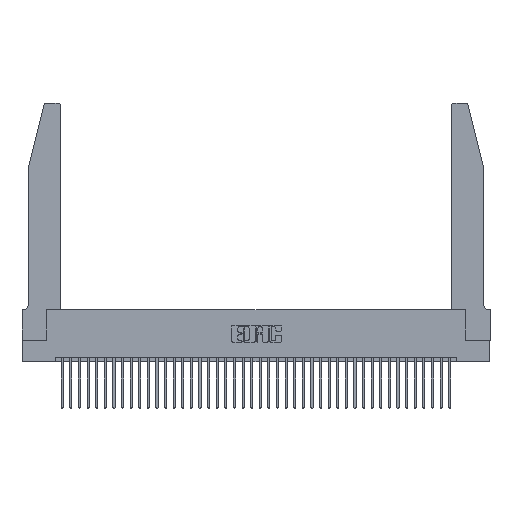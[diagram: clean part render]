
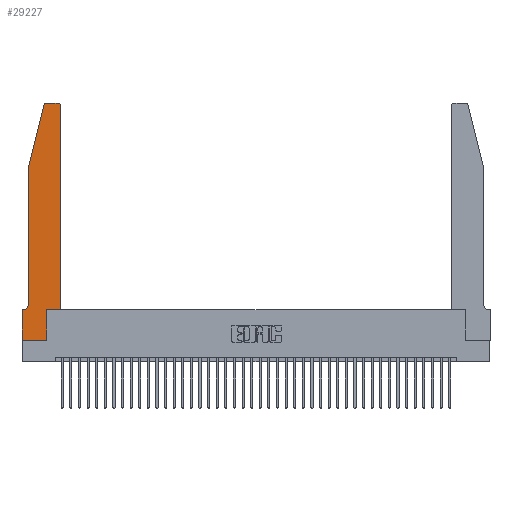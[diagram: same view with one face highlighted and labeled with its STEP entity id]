
A CAD part, top view. The second image highlights one B-rep face of the part: STEP entity #29227.
In plain terms, the highlighted planar face has unit normal (0, 0, 1).
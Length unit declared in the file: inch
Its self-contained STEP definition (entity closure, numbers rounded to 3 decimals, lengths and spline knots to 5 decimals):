
#14 = FACE_OUTER_BOUND ( 'NONE', #1911, .T. ) ;
#633 = VERTEX_POINT ( 'NONE', #12016 ) ;
#730 = LINE ( 'NONE', #8545, #3684 ) ;
#1793 = CARTESIAN_POINT ( 'NONE',  ( 0., 0.35, 0.37 ) ) ;
#1911 = EDGE_LOOP ( 'NONE', ( #19973, #6507, #27655, #17372, #18773, #4992, #32163, #4681, #7863, #10781, #23679, #24845 ) ) ;
#2410 = EDGE_CURVE ( 'NONE', #22411, #9083, #5865, .T. ) ;
#2570 = LINE ( 'NONE', #5586, #18196 ) ;
#2900 = DIRECTION ( 'NONE',  ( 1., 0., 0. ) ) ;
#3074 = CARTESIAN_POINT ( 'NONE',  ( 0., 0., 0.37 ) ) ;
#3684 = VECTOR ( 'NONE', #17501, 39.37008 ) ;
#4178 = VECTOR ( 'NONE', #9894, 39.37008 ) ;
#4681 = ORIENTED_EDGE ( 'NONE', *, *, #6744, .T. ) ;
#4992 = ORIENTED_EDGE ( 'NONE', *, *, #39633, .T. ) ;
#5210 = LINE ( 'NONE', #21528, #19407 ) ;
#5299 = DIRECTION ( 'NONE',  ( 1., 0., 0. ) ) ;
#5563 = VERTEX_POINT ( 'NONE', #37690 ) ;
#5586 = CARTESIAN_POINT ( 'NONE',  ( 0.0755, 2., 0.37 ) ) ;
#5865 = CIRCLE ( 'NONE', #39976, 0.03 ) ;
#6165 = AXIS2_PLACEMENT_3D ( 'NONE', #13944, #20274, #32381 ) ;
#6414 = DIRECTION ( 'NONE',  ( 0., -1., 0. ) ) ;
#6507 = ORIENTED_EDGE ( 'NONE', *, *, #2410, .T. ) ;
#6744 = EDGE_CURVE ( 'NONE', #34862, #34130, #36889, .T. ) ;
#6835 = DIRECTION ( 'NONE',  ( 0., 1., 0. ) ) ;
#7863 = ORIENTED_EDGE ( 'NONE', *, *, #10081, .T. ) ;
#8545 = CARTESIAN_POINT ( 'NONE',  ( 0.2605, 2.75, 0.37 ) ) ;
#8642 = LINE ( 'NONE', #22386, #4178 ) ;
#9083 = VERTEX_POINT ( 'NONE', #35596 ) ;
#9228 = DIRECTION ( 'NONE',  ( 0., 0., -1. ) ) ;
#9268 = VECTOR ( 'NONE', #23286, 39.37008 ) ;
#9735 = LINE ( 'NONE', #20168, #9268 ) ;
#9871 = AXIS2_PLACEMENT_3D ( 'NONE', #21584, #9228, #31115 ) ;
#9894 = DIRECTION ( 'NONE',  ( -1., 0., 0. ) ) ;
#10081 = EDGE_CURVE ( 'NONE', #34130, #5563, #20581, .T. ) ;
#10600 = EDGE_CURVE ( 'NONE', #23620, #11695, #31735, .T. ) ;
#10781 = ORIENTED_EDGE ( 'NONE', *, *, #31041, .T. ) ;
#11695 = VERTEX_POINT ( 'NONE', #23005 ) ;
#12016 = CARTESIAN_POINT ( 'NONE',  ( 0.4505, 0.35, 0.37 ) ) ;
#12352 = VECTOR ( 'NONE', #6414, 39.37008 ) ;
#13161 = EDGE_CURVE ( 'NONE', #16193, #29818, #15957, .T. ) ;
#13944 = CARTESIAN_POINT ( 'NONE',  ( 0.4205, 2.72, 0.37 ) ) ;
#15643 = LINE ( 'NONE', #35319, #24914 ) ;
#15957 = CIRCLE ( 'NONE', #9871, 0.07 ) ;
#16193 = VERTEX_POINT ( 'NONE', #22624 ) ;
#17169 = VECTOR ( 'NONE', #20686, 39.37008 ) ;
#17337 = VERTEX_POINT ( 'NONE', #29270 ) ;
#17372 = ORIENTED_EDGE ( 'NONE', *, *, #22226, .T. ) ;
#17501 = DIRECTION ( 'NONE',  ( -1., 0., 0. ) ) ;
#18196 = VECTOR ( 'NONE', #36110, 39.37008 ) ;
#18749 = CARTESIAN_POINT ( 'NONE',  ( 0.0755, 2., 0.37 ) ) ;
#18773 = ORIENTED_EDGE ( 'NONE', *, *, #13161, .T. ) ;
#19304 = VERTEX_POINT ( 'NONE', #24034 ) ;
#19407 = VECTOR ( 'NONE', #25040, 39.37008 ) ;
#19973 = ORIENTED_EDGE ( 'NONE', *, *, #31986, .T. ) ;
#20168 = CARTESIAN_POINT ( 'NONE',  ( 0., 0., 0.37 ) ) ;
#20274 = DIRECTION ( 'NONE',  ( 0., 0., 1. ) ) ;
#20581 = LINE ( 'NONE', #23662, #17169 ) ;
#20686 = DIRECTION ( 'NONE',  ( 0., 1., 0. ) ) ;
#20884 = PLANE ( 'NONE',  #21546 ) ;
#21528 = CARTESIAN_POINT ( 'NONE',  ( 0.4505, 0.35, 0.37 ) ) ;
#21546 = AXIS2_PLACEMENT_3D ( 'NONE', #1793, #23592, #5299 ) ;
#21584 = CARTESIAN_POINT ( 'NONE',  ( 0.0055, 0.42, 0.37 ) ) ;
#22226 = EDGE_CURVE ( 'NONE', #19304, #16193, #38695, .T. ) ;
#22386 = CARTESIAN_POINT ( 'NONE',  ( 0.0755, 0.35, 0.37 ) ) ;
#22411 = VERTEX_POINT ( 'NONE', #23031 ) ;
#22624 = CARTESIAN_POINT ( 'NONE',  ( 0.0755, 0.42, 0.37 ) ) ;
#23005 = CARTESIAN_POINT ( 'NONE',  ( 0.4205, 2.75, 0.37 ) ) ;
#23031 = CARTESIAN_POINT ( 'NONE',  ( 0.284, 2.75, 0.37 ) ) ;
#23286 = DIRECTION ( 'NONE',  ( 0., -1., 0. ) ) ;
#23592 = DIRECTION ( 'NONE',  ( 0., 0., 1. ) ) ;
#23620 = VERTEX_POINT ( 'NONE', #31791 ) ;
#23662 = CARTESIAN_POINT ( 'NONE',  ( 0.2865, 0.35, 0.37 ) ) ;
#23679 = ORIENTED_EDGE ( 'NONE', *, *, #28914, .T. ) ;
#24034 = CARTESIAN_POINT ( 'NONE',  ( 0.0755, 2., 0.37 ) ) ;
#24710 = VECTOR ( 'NONE', #2900, 39.37008 ) ;
#24845 = ORIENTED_EDGE ( 'NONE', *, *, #10600, .T. ) ;
#24914 = VECTOR ( 'NONE', #6835, 39.37008 ) ;
#24930 = CARTESIAN_POINT ( 'NONE',  ( 0.284, 2.72, 0.37 ) ) ;
#25040 = DIRECTION ( 'NONE',  ( 1., 0., 0. ) ) ;
#27372 = EDGE_CURVE ( 'NONE', #9083, #19304, #2570, .T. ) ;
#27655 = ORIENTED_EDGE ( 'NONE', *, *, #27372, .T. ) ;
#27908 = EDGE_CURVE ( 'NONE', #17337, #34862, #9735, .T. ) ;
#28914 = EDGE_CURVE ( 'NONE', #633, #23620, #15643, .T. ) ;
#29227 = ADVANCED_FACE ( 'NONE', ( #14 ), #20884, .T. ) ;
#29270 = CARTESIAN_POINT ( 'NONE',  ( 0., 0.35, 0.37 ) ) ;
#29818 = VERTEX_POINT ( 'NONE', #30345 ) ;
#30345 = CARTESIAN_POINT ( 'NONE',  ( 0.0055, 0.35, 0.37 ) ) ;
#31041 = EDGE_CURVE ( 'NONE', #5563, #633, #5210, .T. ) ;
#31055 = CARTESIAN_POINT ( 'NONE',  ( 0.2865, 0., 0.37 ) ) ;
#31115 = DIRECTION ( 'NONE',  ( -1., 0., 0. ) ) ;
#31735 = CIRCLE ( 'NONE', #6165, 0.03 ) ;
#31791 = CARTESIAN_POINT ( 'NONE',  ( 0.4505, 2.72, 0.37 ) ) ;
#31986 = EDGE_CURVE ( 'NONE', #11695, #22411, #730, .T. ) ;
#32163 = ORIENTED_EDGE ( 'NONE', *, *, #27908, .T. ) ;
#32381 = DIRECTION ( 'NONE',  ( 1., 0., 0. ) ) ;
#34130 = VERTEX_POINT ( 'NONE', #31055 ) ;
#34485 = CARTESIAN_POINT ( 'NONE',  ( 0., 0., 0.37 ) ) ;
#34862 = VERTEX_POINT ( 'NONE', #3074 ) ;
#35319 = CARTESIAN_POINT ( 'NONE',  ( 0.4505, 0.35, 0.37 ) ) ;
#35596 = CARTESIAN_POINT ( 'NONE',  ( 0.25487, 2.72718, 0.37 ) ) ;
#36110 = DIRECTION ( 'NONE',  ( -0.239, -0.971, 0. ) ) ;
#36889 = LINE ( 'NONE', #34485, #24710 ) ;
#37191 = DIRECTION ( 'NONE',  ( 1., 0., 0. ) ) ;
#37690 = CARTESIAN_POINT ( 'NONE',  ( 0.2865, 0.35, 0.37 ) ) ;
#38695 = LINE ( 'NONE', #18749, #12352 ) ;
#39633 = EDGE_CURVE ( 'NONE', #29818, #17337, #8642, .T. ) ;
#39976 = AXIS2_PLACEMENT_3D ( 'NONE', #24930, #40355, #37191 ) ;
#40355 = DIRECTION ( 'NONE',  ( 0., 0., 1. ) ) ;
